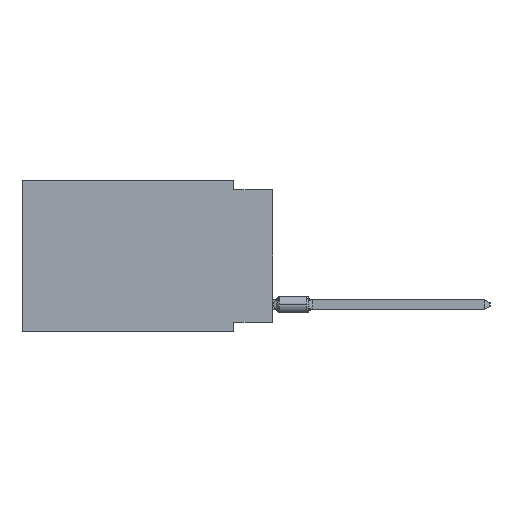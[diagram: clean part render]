
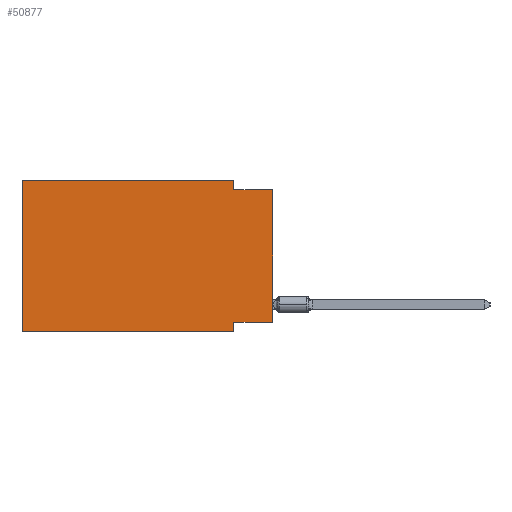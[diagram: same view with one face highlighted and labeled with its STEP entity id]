
A CAD part, left-side view. The second image highlights one B-rep face of the part: STEP entity #50877.
In plain terms, the highlighted planar face has unit normal (-1, 0, 0).
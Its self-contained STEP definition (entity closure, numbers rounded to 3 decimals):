
#395 = VECTOR ( 'NONE', #30978, 1000. ) ;
#1334 = EDGE_CURVE ( 'NONE', #12727, #23594, #23186, .T. ) ;
#1420 = ORIENTED_EDGE ( 'NONE', *, *, #28263, .F. ) ;
#3257 = AXIS2_PLACEMENT_3D ( 'NONE', #38006, #14742, #50150 ) ;
#3774 = CARTESIAN_POINT ( 'NONE',  ( 0., 0., -0.635 ) ) ;
#3904 = CARTESIAN_POINT ( 'NONE',  ( 0., 16.383, 0. ) ) ;
#4430 = LINE ( 'NONE', #32873, #40673 ) ;
#6451 = CARTESIAN_POINT ( 'NONE',  ( 0., 2.54, -9.906 ) ) ;
#7626 = CARTESIAN_POINT ( 'NONE',  ( 0., 2.54, 0. ) ) ;
#8444 = EDGE_CURVE ( 'NONE', #21298, #18749, #26739, .T. ) ;
#8647 = VECTOR ( 'NONE', #49798, 1000. ) ;
#8833 = VECTOR ( 'NONE', #13704, 1000. ) ;
#9097 = ORIENTED_EDGE ( 'NONE', *, *, #28595, .F. ) ;
#9331 = DIRECTION ( 'NONE',  ( 0., -1., 0. ) ) ;
#9947 = VERTEX_POINT ( 'NONE', #45937 ) ;
#10425 = DIRECTION ( 'NONE',  ( 0., 1., 0. ) ) ;
#12727 = VERTEX_POINT ( 'NONE', #30357 ) ;
#13019 = ORIENTED_EDGE ( 'NONE', *, *, #34751, .T. ) ;
#13343 = LINE ( 'NONE', #13865, #8647 ) ;
#13584 = ORIENTED_EDGE ( 'NONE', *, *, #42580, .F. ) ;
#13704 = DIRECTION ( 'NONE',  ( 0., 0., -1. ) ) ;
#13865 = CARTESIAN_POINT ( 'NONE',  ( 0., 2.54, 0. ) ) ;
#13932 = VERTEX_POINT ( 'NONE', #7626 ) ;
#14742 = DIRECTION ( 'NONE',  ( 1., 0., 0. ) ) ;
#15192 = LINE ( 'NONE', #27081, #395 ) ;
#18066 = EDGE_CURVE ( 'NONE', #39783, #23934, #4430, .T. ) ;
#18749 = VERTEX_POINT ( 'NONE', #21046 ) ;
#18799 = DIRECTION ( 'NONE',  ( 0., -1., 0. ) ) ;
#19407 = VECTOR ( 'NONE', #18799, 1000. ) ;
#20308 = ORIENTED_EDGE ( 'NONE', *, *, #8444, .F. ) ;
#21046 = CARTESIAN_POINT ( 'NONE',  ( 0., 2.54, -9.271 ) ) ;
#21298 = VERTEX_POINT ( 'NONE', #49281 ) ;
#22219 = VECTOR ( 'NONE', #49454, 1000. ) ;
#23186 = LINE ( 'NONE', #3774, #19407 ) ;
#23594 = VERTEX_POINT ( 'NONE', #26955 ) ;
#23934 = VERTEX_POINT ( 'NONE', #42421 ) ;
#26130 = LINE ( 'NONE', #6451, #8833 ) ;
#26696 = DIRECTION ( 'NONE',  ( 0., 0., 1. ) ) ;
#26739 = LINE ( 'NONE', #45620, #41851 ) ;
#26955 = CARTESIAN_POINT ( 'NONE',  ( 0., 0., -0.635 ) ) ;
#27081 = CARTESIAN_POINT ( 'NONE',  ( 0., 0., 0. ) ) ;
#27226 = CARTESIAN_POINT ( 'NONE',  ( 0., 16.383, -9.906 ) ) ;
#28263 = EDGE_CURVE ( 'NONE', #39783, #9947, #47352, .T. ) ;
#28595 = EDGE_CURVE ( 'NONE', #18749, #23934, #26130, .T. ) ;
#30357 = CARTESIAN_POINT ( 'NONE',  ( 0., 2.54, -0.635 ) ) ;
#30978 = DIRECTION ( 'NONE',  ( 0., 0., 1. ) ) ;
#32873 = CARTESIAN_POINT ( 'NONE',  ( 0., 16.383, -9.906 ) ) ;
#33032 = ORIENTED_EDGE ( 'NONE', *, *, #40338, .F. ) ;
#34751 = EDGE_CURVE ( 'NONE', #21298, #23594, #15192, .T. ) ;
#37505 = FACE_OUTER_BOUND ( 'NONE', #46854, .T. ) ;
#37958 = ORIENTED_EDGE ( 'NONE', *, *, #1334, .F. ) ;
#38006 = CARTESIAN_POINT ( 'NONE',  ( 0., 16.383, 0. ) ) ;
#39783 = VERTEX_POINT ( 'NONE', #27226 ) ;
#39796 = ORIENTED_EDGE ( 'NONE', *, *, #18066, .T. ) ;
#40338 = EDGE_CURVE ( 'NONE', #13932, #12727, #13343, .T. ) ;
#40673 = VECTOR ( 'NONE', #9331, 1000. ) ;
#41851 = VECTOR ( 'NONE', #10425, 1000. ) ;
#41959 = LINE ( 'NONE', #49194, #22219 ) ;
#42421 = CARTESIAN_POINT ( 'NONE',  ( 0., 2.54, -9.906 ) ) ;
#42580 = EDGE_CURVE ( 'NONE', #9947, #13932, #41959, .T. ) ;
#45198 = VECTOR ( 'NONE', #26696, 1000. ) ;
#45620 = CARTESIAN_POINT ( 'NONE',  ( 0., 0., -9.271 ) ) ;
#45937 = CARTESIAN_POINT ( 'NONE',  ( 0., 16.383, 0. ) ) ;
#46854 = EDGE_LOOP ( 'NONE', ( #13019, #37958, #33032, #13584, #1420, #39796, #9097, #20308 ) ) ;
#47352 = LINE ( 'NONE', #3904, #45198 ) ;
#49194 = CARTESIAN_POINT ( 'NONE',  ( 0., 16.383, 0. ) ) ;
#49281 = CARTESIAN_POINT ( 'NONE',  ( 0., 0., -9.271 ) ) ;
#49390 = PLANE ( 'NONE',  #3257 ) ;
#49454 = DIRECTION ( 'NONE',  ( 0., -1., 0. ) ) ;
#49798 = DIRECTION ( 'NONE',  ( 0., 0., -1. ) ) ;
#50150 = DIRECTION ( 'NONE',  ( 0., 0., -1. ) ) ;
#50877 = ADVANCED_FACE ( 'NONE', ( #37505 ), #49390, .F. ) ;
